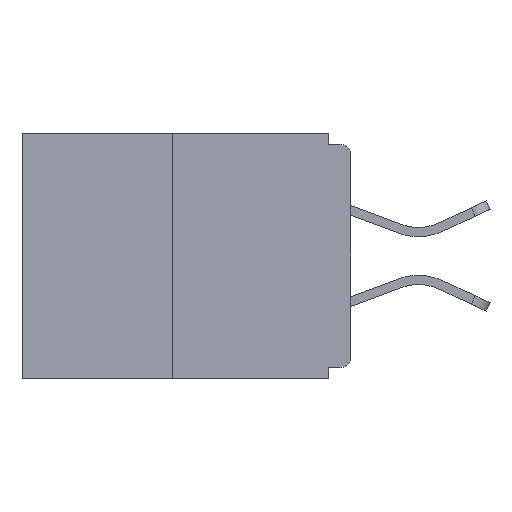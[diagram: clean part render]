
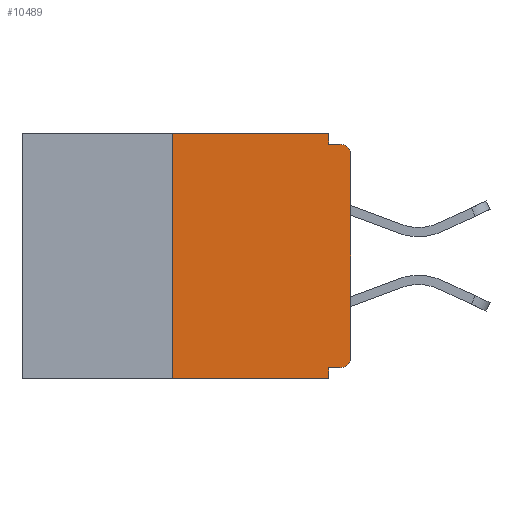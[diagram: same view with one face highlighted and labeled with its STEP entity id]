
A CAD part, left-side view. The second image highlights one B-rep face of the part: STEP entity #10489.
In plain terms, the highlighted planar face has unit normal (-1, 0, 0).
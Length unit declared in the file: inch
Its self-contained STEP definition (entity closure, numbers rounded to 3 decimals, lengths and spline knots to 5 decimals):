
#446 = DIRECTION ( 'NONE',  ( 0., 0., 1. ) ) ;
#726 = CARTESIAN_POINT ( 'NONE',  ( 0., 0.25, 0. ) ) ;
#926 = LINE ( 'NONE', #11372, #5210 ) ;
#979 = LINE ( 'NONE', #2194, #6238 ) ;
#1042 = ORIENTED_EDGE ( 'NONE', *, *, #1226, .T. ) ;
#1217 = ORIENTED_EDGE ( 'NONE', *, *, #13644, .T. ) ;
#1226 = EDGE_CURVE ( 'NONE', #1797, #6647, #14026, .T. ) ;
#1246 = CARTESIAN_POINT ( 'NONE',  ( 0., 0.015, -0.313 ) ) ;
#1255 = LINE ( 'NONE', #9181, #10355 ) ;
#1353 = VECTOR ( 'NONE', #9372, 39.37008 ) ;
#1409 = CARTESIAN_POINT ( 'NONE',  ( 0., 0., -0.313 ) ) ;
#1528 = VERTEX_POINT ( 'NONE', #6395 ) ;
#1690 = EDGE_CURVE ( 'NONE', #3728, #10472, #5357, .T. ) ;
#1797 = VERTEX_POINT ( 'NONE', #12678 ) ;
#1994 = EDGE_CURVE ( 'NONE', #11330, #14273, #13249, .T. ) ;
#2107 = AXIS2_PLACEMENT_3D ( 'NONE', #9107, #5828, #8756 ) ;
#2157 = DIRECTION ( 'NONE',  ( 0., -1., 0. ) ) ;
#2194 = CARTESIAN_POINT ( 'NONE',  ( 0., 0.46, 0. ) ) ;
#2197 = EDGE_CURVE ( 'NONE', #13698, #14273, #8385, .T. ) ;
#2239 = EDGE_CURVE ( 'NONE', #3454, #11330, #926, .T. ) ;
#2285 = EDGE_CURVE ( 'NONE', #1528, #8405, #1255, .T. ) ;
#2568 = ORIENTED_EDGE ( 'NONE', *, *, #2239, .F. ) ;
#2783 = VECTOR ( 'NONE', #446, 39.37008 ) ;
#2856 = EDGE_CURVE ( 'NONE', #3728, #8405, #4927, .T. ) ;
#3067 = VECTOR ( 'NONE', #8511, 39.37008 ) ;
#3139 = DIRECTION ( 'NONE',  ( 0., 0., -1. ) ) ;
#3239 = ORIENTED_EDGE ( 'NONE', *, *, #2285, .F. ) ;
#3248 = CARTESIAN_POINT ( 'NONE',  ( 0., 0., -0.03 ) ) ;
#3452 = CARTESIAN_POINT ( 'NONE',  ( 0., 0.25, 0. ) ) ;
#3454 = VERTEX_POINT ( 'NONE', #11852 ) ;
#3469 = DIRECTION ( 'NONE',  ( -1., 0., 0. ) ) ;
#3536 = DIRECTION ( 'NONE',  ( 1., 0., 0. ) ) ;
#3728 = VERTEX_POINT ( 'NONE', #13689 ) ;
#3981 = EDGE_CURVE ( 'NONE', #10472, #3454, #979, .T. ) ;
#4256 = EDGE_LOOP ( 'NONE', ( #11774, #6871, #13345, #3239, #13919, #1042, #1217, #6083, #7517, #2568 ) ) ;
#4329 = CARTESIAN_POINT ( 'NONE',  ( 0., 0., -0.015 ) ) ;
#4690 = LINE ( 'NONE', #4912, #1353 ) ;
#4710 = FACE_OUTER_BOUND ( 'NONE', #4256, .T. ) ;
#4908 = AXIS2_PLACEMENT_3D ( 'NONE', #1246, #3469, #5371 ) ;
#4912 = CARTESIAN_POINT ( 'NONE',  ( 0., 0., -0.328 ) ) ;
#4927 = LINE ( 'NONE', #12826, #8509 ) ;
#5210 = VECTOR ( 'NONE', #3139, 39.37008 ) ;
#5357 = LINE ( 'NONE', #3452, #2783 ) ;
#5371 = DIRECTION ( 'NONE',  ( 0., 0., -1. ) ) ;
#5725 = EDGE_CURVE ( 'NONE', #1797, #1528, #4690, .T. ) ;
#5828 = DIRECTION ( 'NONE',  ( -1., 0., 0. ) ) ;
#6038 = DIRECTION ( 'NONE',  ( 0., -1., 0. ) ) ;
#6083 = ORIENTED_EDGE ( 'NONE', *, *, #2197, .T. ) ;
#6238 = VECTOR ( 'NONE', #12322, 39.37008 ) ;
#6395 = CARTESIAN_POINT ( 'NONE',  ( 0., 0.031, -0.328 ) ) ;
#6647 = VERTEX_POINT ( 'NONE', #1409 ) ;
#6871 = ORIENTED_EDGE ( 'NONE', *, *, #1690, .F. ) ;
#7517 = ORIENTED_EDGE ( 'NONE', *, *, #1994, .F. ) ;
#7896 = CARTESIAN_POINT ( 'NONE',  ( 0., 0.031, -0.343 ) ) ;
#8342 = PLANE ( 'NONE',  #10701 ) ;
#8385 = CIRCLE ( 'NONE', #2107, 0.015 ) ;
#8405 = VERTEX_POINT ( 'NONE', #7896 ) ;
#8509 = VECTOR ( 'NONE', #6038, 39.37008 ) ;
#8511 = DIRECTION ( 'NONE',  ( 0., 0., 1. ) ) ;
#8632 = CARTESIAN_POINT ( 'NONE',  ( 0., 0.015, -0.015 ) ) ;
#8756 = DIRECTION ( 'NONE',  ( 0., 0., -1. ) ) ;
#9107 = CARTESIAN_POINT ( 'NONE',  ( 0., 0.015, -0.03 ) ) ;
#9181 = CARTESIAN_POINT ( 'NONE',  ( 0., 0.031, -0.343 ) ) ;
#9372 = DIRECTION ( 'NONE',  ( 0., 1., 0. ) ) ;
#10184 = CARTESIAN_POINT ( 'NONE',  ( 0., 0.46, 0. ) ) ;
#10355 = VECTOR ( 'NONE', #14284, 39.37008 ) ;
#10472 = VERTEX_POINT ( 'NONE', #726 ) ;
#10489 = ADVANCED_FACE ( 'NONE', ( #4710 ), #8342, .F. ) ;
#10701 = AXIS2_PLACEMENT_3D ( 'NONE', #10184, #3536, #11632 ) ;
#11330 = VERTEX_POINT ( 'NONE', #11373 ) ;
#11372 = CARTESIAN_POINT ( 'NONE',  ( 0., 0.031, 0. ) ) ;
#11373 = CARTESIAN_POINT ( 'NONE',  ( 0., 0.031, -0.015 ) ) ;
#11632 = DIRECTION ( 'NONE',  ( 0., 0., -1. ) ) ;
#11655 = VECTOR ( 'NONE', #2157, 39.37008 ) ;
#11774 = ORIENTED_EDGE ( 'NONE', *, *, #3981, .F. ) ;
#11852 = CARTESIAN_POINT ( 'NONE',  ( 0., 0.031, 0. ) ) ;
#12322 = DIRECTION ( 'NONE',  ( 0., -1., 0. ) ) ;
#12678 = CARTESIAN_POINT ( 'NONE',  ( 0., 0.015, -0.328 ) ) ;
#12826 = CARTESIAN_POINT ( 'NONE',  ( 0., 0.46, -0.343 ) ) ;
#13249 = LINE ( 'NONE', #4329, #11655 ) ;
#13345 = ORIENTED_EDGE ( 'NONE', *, *, #2856, .T. ) ;
#13644 = EDGE_CURVE ( 'NONE', #6647, #13698, #14096, .T. ) ;
#13689 = CARTESIAN_POINT ( 'NONE',  ( 0., 0.25, -0.343 ) ) ;
#13698 = VERTEX_POINT ( 'NONE', #3248 ) ;
#13919 = ORIENTED_EDGE ( 'NONE', *, *, #5725, .F. ) ;
#14026 = CIRCLE ( 'NONE', #4908, 0.015 ) ;
#14096 = LINE ( 'NONE', #14167, #3067 ) ;
#14167 = CARTESIAN_POINT ( 'NONE',  ( 0., 0., 0. ) ) ;
#14273 = VERTEX_POINT ( 'NONE', #8632 ) ;
#14284 = DIRECTION ( 'NONE',  ( 0., 0., -1. ) ) ;
